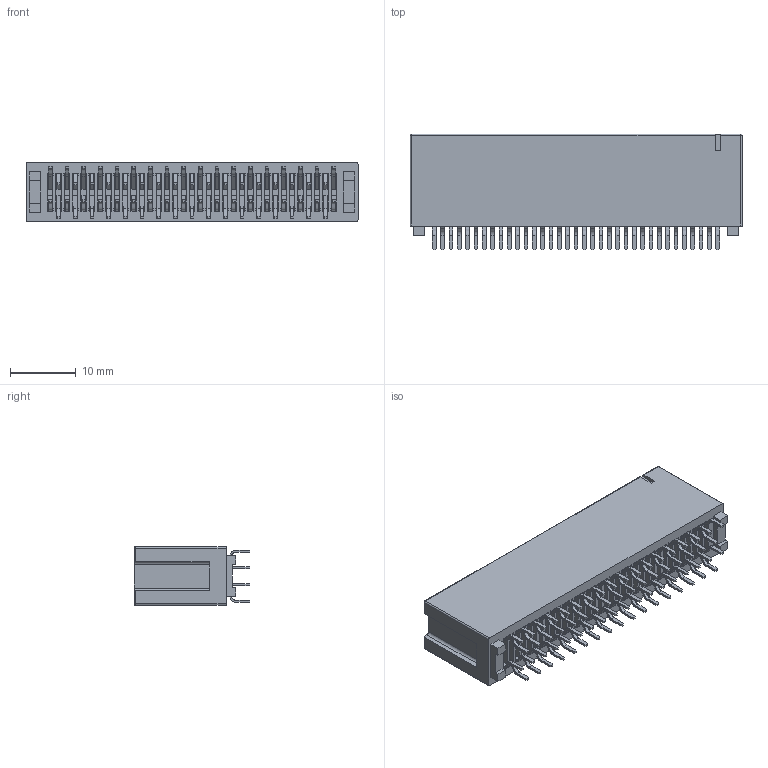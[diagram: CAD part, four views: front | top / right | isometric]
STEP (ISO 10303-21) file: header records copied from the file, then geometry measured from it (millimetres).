
FILE_DESCRIPTION (( 'STEP AP203' ), '1' );
FILE_NAME ('302-070-221-201.STEP', '2024-04-01T19:32:29', ( '' ), ( '' ), 'SwSTEP 2.0', 'SolidWorks 2023', '' );
FILE_SCHEMA (( 'CONFIG_CONTROL_DESIGN' ));
Length unit declared in the file: millimetre
Products named in the file (4): 302-070-221-201; HSG_Vertical HSG; Contact_302-290-X21 (2); Contact_302-290-X21 (1)
Assembly tree (71 placements, depth 2):
  302-070-221-201
    HSG_Vertical HSG
    Contact_302-290-X21 (2)  x35
    Contact_302-290-X21 (1)  x35
Bounding box: 50.55 x 17.63 x 8.88 mm (x, y, z)
Volume: 3929.3 mm3; surface area: 10747.8 mm2
Topology: 71 solids, 71 shells, 3251 faces, 9548 edges, 6264 vertices
Faces by surface type: plane 2394, cylinder 713, bspline 140, sphere 4
Entity records: 28886 total; most frequent: CARTESIAN_POINT 4957, ORIENTED_EDGE 4944, DIRECTION 4004, EDGE_CURVE 2472, VECTOR 2398, LINE 2398, VERTEX_POINT 1640, AXIS2_PLACEMENT_3D 803
